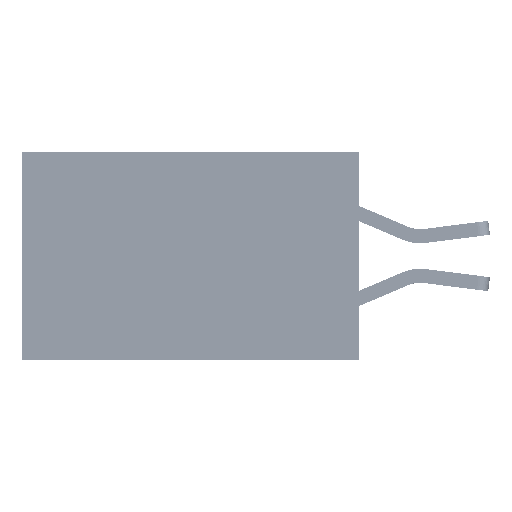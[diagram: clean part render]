
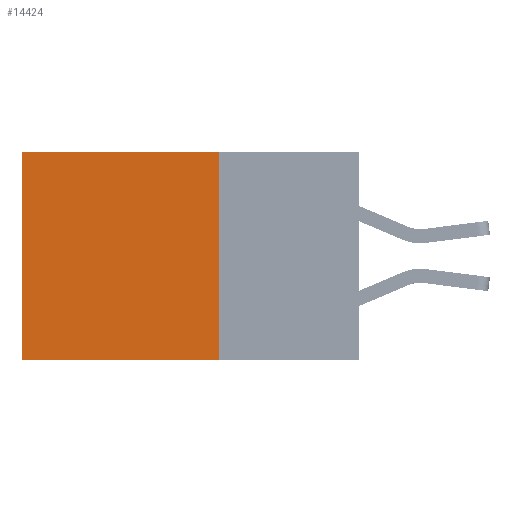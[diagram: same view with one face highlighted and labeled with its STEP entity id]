
A CAD part, left-side view. The second image highlights one B-rep face of the part: STEP entity #14424.
In plain terms, the highlighted planar face has unit normal (-1, 0, 0).
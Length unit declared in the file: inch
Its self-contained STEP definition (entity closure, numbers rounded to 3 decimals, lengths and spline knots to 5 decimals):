
#804 = VECTOR ( 'NONE', #45228, 39.37008 ) ;
#3294 = DIRECTION ( 'NONE',  ( 0., 0., -1. ) ) ;
#4440 = DIRECTION ( 'NONE',  ( 0., 0., -1. ) ) ;
#7622 = VERTEX_POINT ( 'NONE', #15014 ) ;
#7667 = DIRECTION ( 'NONE',  ( 0., 1., 0. ) ) ;
#8280 = LINE ( 'NONE', #11386, #21733 ) ;
#10720 = EDGE_CURVE ( 'NONE', #35966, #19704, #21908, .T. ) ;
#11381 = VECTOR ( 'NONE', #7667, 39.37008 ) ;
#11386 = CARTESIAN_POINT ( 'NONE',  ( 0.2875, 0.25, 0. ) ) ;
#13041 = CARTESIAN_POINT ( 'NONE',  ( 0.2875, 0.25, 0. ) ) ;
#13055 = ORIENTED_EDGE ( 'NONE', *, *, #21549, .T. ) ;
#14424 = ADVANCED_FACE ( 'NONE', ( #50958 ), #25710, .F. ) ;
#15014 = CARTESIAN_POINT ( 'NONE',  ( 0.2875, 0.25, 0. ) ) ;
#16791 = ORIENTED_EDGE ( 'NONE', *, *, #19836, .T. ) ;
#18020 = ORIENTED_EDGE ( 'NONE', *, *, #10720, .F. ) ;
#19494 = CARTESIAN_POINT ( 'NONE',  ( 0.2875, 0.25, -0.37 ) ) ;
#19704 = VERTEX_POINT ( 'NONE', #35780 ) ;
#19707 = LINE ( 'NONE', #39963, #11381 ) ;
#19836 = EDGE_CURVE ( 'NONE', #41468, #19704, #24405, .T. ) ;
#21549 = EDGE_CURVE ( 'NONE', #7622, #41468, #19707, .T. ) ;
#21733 = VECTOR ( 'NONE', #3294, 39.37008 ) ;
#21908 = LINE ( 'NONE', #52539, #804 ) ;
#24380 = CARTESIAN_POINT ( 'NONE',  ( 0.2875, 0.6, 0. ) ) ;
#24405 = LINE ( 'NONE', #24380, #37765 ) ;
#25710 = PLANE ( 'NONE',  #30122 ) ;
#26697 = ORIENTED_EDGE ( 'NONE', *, *, #35464, .F. ) ;
#28925 = DIRECTION ( 'NONE',  ( 1., 0., 0. ) ) ;
#30122 = AXIS2_PLACEMENT_3D ( 'NONE', #13041, #28925, #4440 ) ;
#31558 = CARTESIAN_POINT ( 'NONE',  ( 0.2875, 0.6, 0. ) ) ;
#32030 = DIRECTION ( 'NONE',  ( 0., 0., -1. ) ) ;
#35464 = EDGE_CURVE ( 'NONE', #7622, #35966, #8280, .T. ) ;
#35780 = CARTESIAN_POINT ( 'NONE',  ( 0.2875, 0.6, -0.37 ) ) ;
#35966 = VERTEX_POINT ( 'NONE', #19494 ) ;
#36988 = EDGE_LOOP ( 'NONE', ( #16791, #18020, #26697, #13055 ) ) ;
#37765 = VECTOR ( 'NONE', #32030, 39.37008 ) ;
#39963 = CARTESIAN_POINT ( 'NONE',  ( 0.2875, 0.25, 0. ) ) ;
#41468 = VERTEX_POINT ( 'NONE', #31558 ) ;
#45228 = DIRECTION ( 'NONE',  ( 0., 1., 0. ) ) ;
#50958 = FACE_OUTER_BOUND ( 'NONE', #36988, .T. ) ;
#52539 = CARTESIAN_POINT ( 'NONE',  ( 0.2875, 0.25, -0.37 ) ) ;
